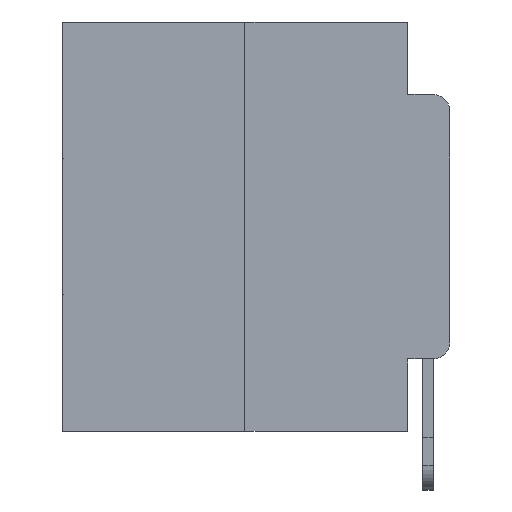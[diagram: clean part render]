
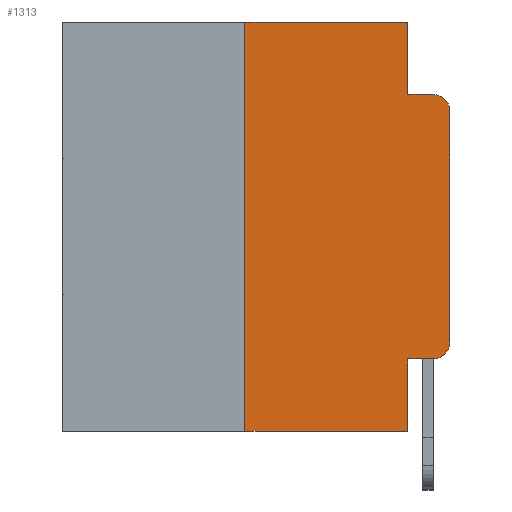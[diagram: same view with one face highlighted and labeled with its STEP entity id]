
A CAD part, left-side view. The second image highlights one B-rep face of the part: STEP entity #1313.
In plain terms, the highlighted planar face has unit normal (-1, 0, 0).
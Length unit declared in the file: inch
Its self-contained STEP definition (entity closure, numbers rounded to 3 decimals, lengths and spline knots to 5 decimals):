
#138 = DIRECTION ( 'NONE',  ( 0., -1., 0. ) ) ;
#628 = VERTEX_POINT ( 'NONE', #6739 ) ;
#673 = VECTOR ( 'NONE', #20645, 39.37008 ) ;
#899 = ORIENTED_EDGE ( 'NONE', *, *, #4887, .F. ) ;
#1313 = ADVANCED_FACE ( 'NONE', ( #22629 ), #12565, .F. ) ;
#1395 = DIRECTION ( 'NONE',  ( 0., 0., 1. ) ) ;
#1489 = CARTESIAN_POINT ( 'NONE',  ( 0., 0.25, 0. ) ) ;
#1531 = CARTESIAN_POINT ( 'NONE',  ( 0., 0.02, -0.1085 ) ) ;
#1691 = EDGE_LOOP ( 'NONE', ( #11639, #27193, #24691, #899, #11192, #5949, #25065, #13542, #12770, #8817 ) ) ;
#2070 = VERTEX_POINT ( 'NONE', #13610 ) ;
#3744 = DIRECTION ( 'NONE',  ( 0., -1., 0. ) ) ;
#3827 = CARTESIAN_POINT ( 'NONE',  ( 0., 0., -0.1085 ) ) ;
#4194 = DIRECTION ( 'NONE',  ( 0., 0., -1. ) ) ;
#4273 = VERTEX_POINT ( 'NONE', #3827 ) ;
#4600 = CARTESIAN_POINT ( 'NONE',  ( 0., 0.02, -0.3915 ) ) ;
#4869 = LINE ( 'NONE', #6791, #24754 ) ;
#4887 = EDGE_CURVE ( 'NONE', #15447, #22398, #15837, .T. ) ;
#5342 = CARTESIAN_POINT ( 'NONE',  ( 0., 0.25, -0.5 ) ) ;
#5473 = VERTEX_POINT ( 'NONE', #25599 ) ;
#5676 = DIRECTION ( 'NONE',  ( 0., 0., -1. ) ) ;
#5747 = CARTESIAN_POINT ( 'NONE',  ( 0., 0.051, 0. ) ) ;
#5949 = ORIENTED_EDGE ( 'NONE', *, *, #13816, .F. ) ;
#6263 = EDGE_CURVE ( 'NONE', #8418, #16803, #8189, .T. ) ;
#6327 = LINE ( 'NONE', #26891, #673 ) ;
#6739 = CARTESIAN_POINT ( 'NONE',  ( 0., 0., -0.3915 ) ) ;
#6791 = CARTESIAN_POINT ( 'NONE',  ( 0., 0.051, -0.4115 ) ) ;
#7036 = CARTESIAN_POINT ( 'NONE',  ( 0., 0.051, -0.0885 ) ) ;
#8189 = LINE ( 'NONE', #27324, #9159 ) ;
#8418 = VERTEX_POINT ( 'NONE', #5342 ) ;
#8464 = EDGE_CURVE ( 'NONE', #628, #4273, #23987, .T. ) ;
#8817 = ORIENTED_EDGE ( 'NONE', *, *, #23868, .T. ) ;
#9159 = VECTOR ( 'NONE', #19159, 39.37008 ) ;
#9205 = CARTESIAN_POINT ( 'NONE',  ( 0., 0.051, -0.5 ) ) ;
#10338 = CARTESIAN_POINT ( 'NONE',  ( 0., 0.02, -0.0885 ) ) ;
#10575 = VECTOR ( 'NONE', #3744, 39.37008 ) ;
#10854 = AXIS2_PLACEMENT_3D ( 'NONE', #19240, #14712, #4194 ) ;
#11192 = ORIENTED_EDGE ( 'NONE', *, *, #24730, .F. ) ;
#11639 = ORIENTED_EDGE ( 'NONE', *, *, #8464, .T. ) ;
#12532 = VECTOR ( 'NONE', #13399, 39.37008 ) ;
#12565 = PLANE ( 'NONE',  #10854 ) ;
#12770 = ORIENTED_EDGE ( 'NONE', *, *, #26781, .T. ) ;
#13399 = DIRECTION ( 'NONE',  ( 0., -1., 0. ) ) ;
#13542 = ORIENTED_EDGE ( 'NONE', *, *, #14518, .F. ) ;
#13610 = CARTESIAN_POINT ( 'NONE',  ( 0., 0.051, -0.4115 ) ) ;
#13626 = LINE ( 'NONE', #1489, #17917 ) ;
#13816 = EDGE_CURVE ( 'NONE', #8418, #5473, #13626, .T. ) ;
#14123 = AXIS2_PLACEMENT_3D ( 'NONE', #1531, #14177, #5676 ) ;
#14177 = DIRECTION ( 'NONE',  ( -1., 0., 0. ) ) ;
#14518 = EDGE_CURVE ( 'NONE', #2070, #16803, #6327, .T. ) ;
#14712 = DIRECTION ( 'NONE',  ( 1., 0., 0. ) ) ;
#15447 = VERTEX_POINT ( 'NONE', #5747 ) ;
#15614 = VERTEX_POINT ( 'NONE', #15667 ) ;
#15667 = CARTESIAN_POINT ( 'NONE',  ( 0., 0.02, -0.4115 ) ) ;
#15837 = LINE ( 'NONE', #23903, #25783 ) ;
#16803 = VERTEX_POINT ( 'NONE', #9205 ) ;
#17904 = CIRCLE ( 'NONE', #18332, 0.02 ) ;
#17917 = VECTOR ( 'NONE', #1395, 39.37008 ) ;
#18332 = AXIS2_PLACEMENT_3D ( 'NONE', #4600, #23616, #25616 ) ;
#19159 = DIRECTION ( 'NONE',  ( 0., -1., 0. ) ) ;
#19240 = CARTESIAN_POINT ( 'NONE',  ( 0., 0.473, 0. ) ) ;
#19737 = VERTEX_POINT ( 'NONE', #10338 ) ;
#20645 = DIRECTION ( 'NONE',  ( 0., 0., -1. ) ) ;
#20899 = CARTESIAN_POINT ( 'NONE',  ( 0., 0.473, 0. ) ) ;
#21017 = EDGE_CURVE ( 'NONE', #22398, #19737, #23479, .T. ) ;
#22385 = VECTOR ( 'NONE', #24406, 39.37008 ) ;
#22398 = VERTEX_POINT ( 'NONE', #26547 ) ;
#22629 = FACE_OUTER_BOUND ( 'NONE', #1691, .T. ) ;
#23479 = LINE ( 'NONE', #7036, #12532 ) ;
#23616 = DIRECTION ( 'NONE',  ( -1., 0., 0. ) ) ;
#23868 = EDGE_CURVE ( 'NONE', #15614, #628, #17904, .T. ) ;
#23903 = CARTESIAN_POINT ( 'NONE',  ( 0., 0.051, 0. ) ) ;
#23987 = LINE ( 'NONE', #24496, #22385 ) ;
#24406 = DIRECTION ( 'NONE',  ( 0., 0., 1. ) ) ;
#24452 = DIRECTION ( 'NONE',  ( 0., 0., -1. ) ) ;
#24496 = CARTESIAN_POINT ( 'NONE',  ( 0., 0., 0. ) ) ;
#24691 = ORIENTED_EDGE ( 'NONE', *, *, #21017, .F. ) ;
#24730 = EDGE_CURVE ( 'NONE', #5473, #15447, #27143, .T. ) ;
#24754 = VECTOR ( 'NONE', #138, 39.37008 ) ;
#25065 = ORIENTED_EDGE ( 'NONE', *, *, #6263, .T. ) ;
#25599 = CARTESIAN_POINT ( 'NONE',  ( 0., 0.25, 0. ) ) ;
#25616 = DIRECTION ( 'NONE',  ( 0., 0., -1. ) ) ;
#25783 = VECTOR ( 'NONE', #24452, 39.37008 ) ;
#25806 = EDGE_CURVE ( 'NONE', #4273, #19737, #27127, .T. ) ;
#26547 = CARTESIAN_POINT ( 'NONE',  ( 0., 0.051, -0.0885 ) ) ;
#26781 = EDGE_CURVE ( 'NONE', #2070, #15614, #4869, .T. ) ;
#26891 = CARTESIAN_POINT ( 'NONE',  ( 0., 0.051, 0. ) ) ;
#27127 = CIRCLE ( 'NONE', #14123, 0.02 ) ;
#27143 = LINE ( 'NONE', #20899, #10575 ) ;
#27193 = ORIENTED_EDGE ( 'NONE', *, *, #25806, .T. ) ;
#27324 = CARTESIAN_POINT ( 'NONE',  ( 0., 0.473, -0.5 ) ) ;
